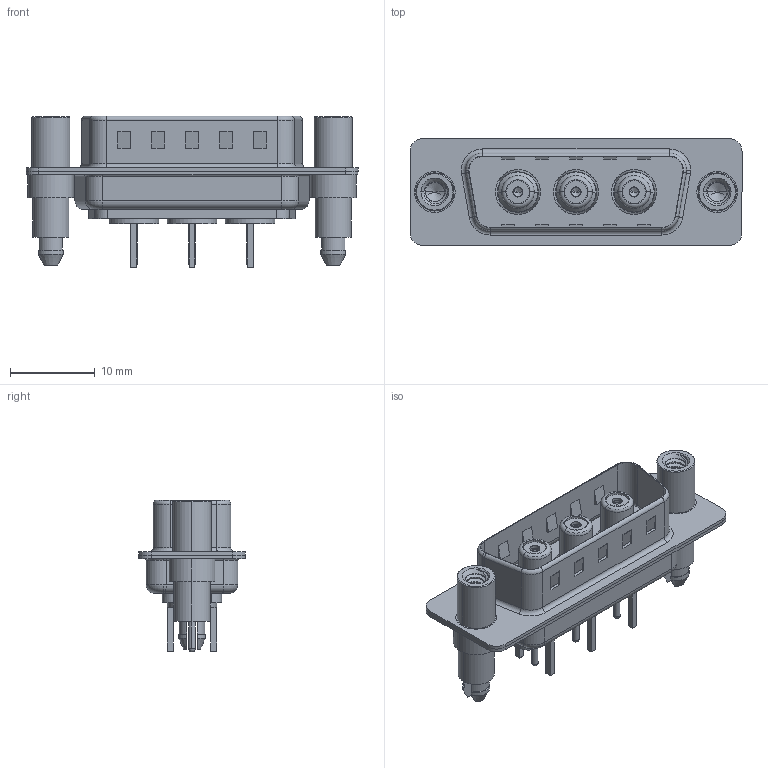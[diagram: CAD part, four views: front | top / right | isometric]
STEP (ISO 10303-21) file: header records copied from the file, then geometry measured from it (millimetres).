
FILE_DESCRIPTION (( 'STEP AP203' ), '1' );
FILE_NAME ('627-3W3-224-5N6.STEP', '2019-05-24T15:14:56', ( '' ), ( '' ), 'SwSTEP 2.0', 'SolidWorks 2016', '' );
FILE_SCHEMA (( 'CONFIG_CONTROL_DESIGN' ));
Length unit declared in the file: millimetre
Products named in the file (11): Insulator Socket 2; Locking Collar; Socket_Str; 627Combo Housing_3W3; Co-Ax Jack Assy_S; 627Combo Shell Rear_15 Contacts; 627-3W3-224-5N6; 627Combo Shell Front_15 Contacts; 627Combo Threaded Standoff and Boardlock_6; Co-Ax Jack_Straight PC Tail; Insulator Socket
Assembly tree (13 placements, depth 3):
  627-3W3-224-5N6
    627Combo Housing_3W3
    627Combo Shell Rear_15 Contacts
    627Combo Shell Front_15 Contacts
    627Combo Threaded Standoff and Boardlock_6  x2
    Co-Ax Jack Assy_S  x3
      Co-Ax Jack_Straight PC Tail
      Insulator Socket
      Insulator Socket 2
      Locking Collar
      Socket_Str
Bounding box: 39.15 x 12.6 x 17.9 mm (x, y, z)
Volume: 2245.9 mm3; surface area: 6388.4 mm2
Topology: 20 solids, 20 shells, 725 faces, 1732 edges, 1088 vertices
Faces by surface type: cylinder 302, plane 298, torus 62, cone 45, bspline 12, sphere 6
Entity records: 15766 total; most frequent: CARTESIAN_POINT 3585, DIRECTION 2394, ORIENTED_EDGE 2210, EDGE_CURVE 1105, AXIS2_PLACEMENT_3D 899, VERTEX_POINT 699, LINE 596, VECTOR 596
